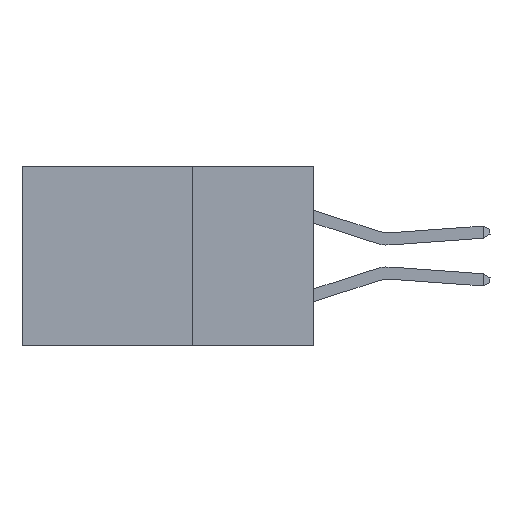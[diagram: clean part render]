
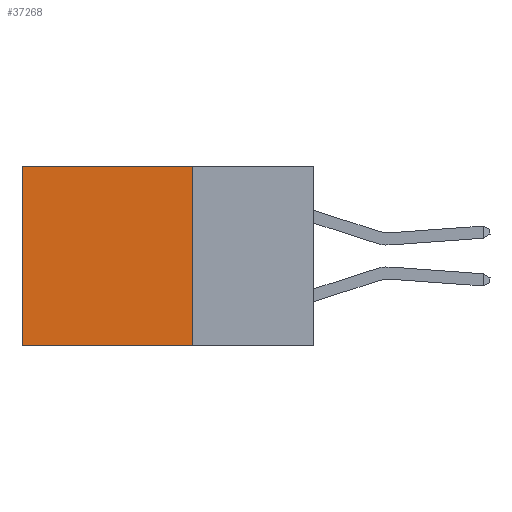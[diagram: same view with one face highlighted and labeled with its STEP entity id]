
A CAD part, left-side view. The second image highlights one B-rep face of the part: STEP entity #37268.
In plain terms, the highlighted planar face has unit normal (-1, 0, 0).
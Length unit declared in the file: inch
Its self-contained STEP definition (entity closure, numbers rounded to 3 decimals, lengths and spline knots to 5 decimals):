
#69 = VECTOR ( 'NONE', #24841, 39.37008 ) ;
#138 = CARTESIAN_POINT ( 'NONE',  ( 0.2875, 0.6, -0.37 ) ) ;
#218 = VECTOR ( 'NONE', #37090, 39.37008 ) ;
#241 = ORIENTED_EDGE ( 'NONE', *, *, #40820, .F. ) ;
#975 = FACE_OUTER_BOUND ( 'NONE', #39115, .T. ) ;
#2241 = AXIS2_PLACEMENT_3D ( 'NONE', #19000, #41146, #22218 ) ;
#2387 = VERTEX_POINT ( 'NONE', #30089 ) ;
#2775 = LINE ( 'NONE', #37781, #36761 ) ;
#5873 = VERTEX_POINT ( 'NONE', #39364 ) ;
#6156 = EDGE_CURVE ( 'NONE', #2387, #20614, #8796, .T. ) ;
#6966 = ORIENTED_EDGE ( 'NONE', *, *, #6156, .F. ) ;
#8796 = LINE ( 'NONE', #34101, #69 ) ;
#14379 = CARTESIAN_POINT ( 'NONE',  ( 0.2875, 0.25, 0. ) ) ;
#14906 = CARTESIAN_POINT ( 'NONE',  ( 0.2875, 0.25, 0. ) ) ;
#19000 = CARTESIAN_POINT ( 'NONE',  ( 0.2875, 0.25, 0. ) ) ;
#20614 = VERTEX_POINT ( 'NONE', #138 ) ;
#22043 = DIRECTION ( 'NONE',  ( 0., 0., -1. ) ) ;
#22218 = DIRECTION ( 'NONE',  ( 0., 0., -1. ) ) ;
#24389 = EDGE_CURVE ( 'NONE', #35541, #5873, #39472, .T. ) ;
#24841 = DIRECTION ( 'NONE',  ( 0., 1., 0. ) ) ;
#25360 = CARTESIAN_POINT ( 'NONE',  ( 0.2875, 0.25, 0. ) ) ;
#27656 = ORIENTED_EDGE ( 'NONE', *, *, #40996, .T. ) ;
#28513 = DIRECTION ( 'NONE',  ( 0., 1., 0. ) ) ;
#30089 = CARTESIAN_POINT ( 'NONE',  ( 0.2875, 0.25, -0.37 ) ) ;
#31064 = VECTOR ( 'NONE', #28513, 39.37008 ) ;
#33304 = LINE ( 'NONE', #14906, #218 ) ;
#34101 = CARTESIAN_POINT ( 'NONE',  ( 0.2875, 0.25, -0.37 ) ) ;
#35541 = VERTEX_POINT ( 'NONE', #14379 ) ;
#36761 = VECTOR ( 'NONE', #22043, 39.37008 ) ;
#37090 = DIRECTION ( 'NONE',  ( 0., 0., -1. ) ) ;
#37100 = ORIENTED_EDGE ( 'NONE', *, *, #24389, .T. ) ;
#37268 = ADVANCED_FACE ( 'NONE', ( #975 ), #37960, .F. ) ;
#37781 = CARTESIAN_POINT ( 'NONE',  ( 0.2875, 0.6, 0. ) ) ;
#37960 = PLANE ( 'NONE',  #2241 ) ;
#39115 = EDGE_LOOP ( 'NONE', ( #27656, #6966, #241, #37100 ) ) ;
#39364 = CARTESIAN_POINT ( 'NONE',  ( 0.2875, 0.6, 0. ) ) ;
#39472 = LINE ( 'NONE', #25360, #31064 ) ;
#40820 = EDGE_CURVE ( 'NONE', #35541, #2387, #33304, .T. ) ;
#40996 = EDGE_CURVE ( 'NONE', #5873, #20614, #2775, .T. ) ;
#41146 = DIRECTION ( 'NONE',  ( 1., 0., 0. ) ) ;
